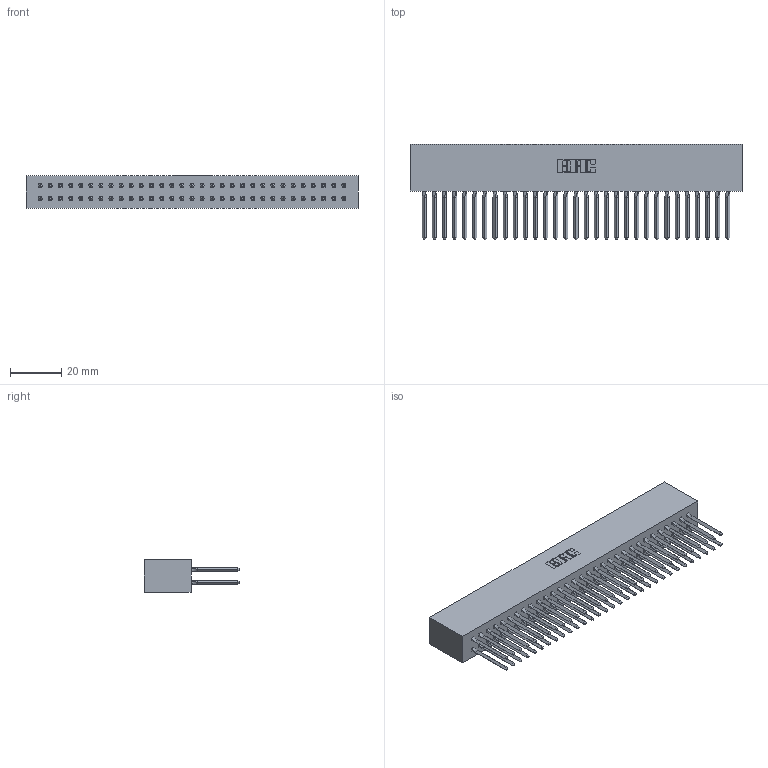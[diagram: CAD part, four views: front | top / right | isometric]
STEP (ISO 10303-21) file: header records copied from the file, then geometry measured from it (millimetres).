
FILE_DESCRIPTION (( 'STEP AP203' ), '1' );
FILE_NAME ('317-062-540-801.STEP', '2020-02-28T05:19:01', ( '' ), ( '' ), 'SwSTEP 2.0', 'SolidWorks 2016', '' );
FILE_SCHEMA (( 'CONFIG_CONTROL_DESIGN' ));
Length unit declared in the file: inch
Products named in the file (3): 317-062-540-801; 317 Part_Lugless; 317-290-001_540
Assembly tree (63 placements, depth 2):
  317-062-540-801
    317 Part_Lugless
    317-290-001_540  x62
Bounding box: 130.05 x 37.34 x 12.7 mm (x, y, z)
Volume: 23247.7 mm3; surface area: 34501.6 mm2
Topology: 63 solids, 63 shells, 5608 faces, 15553 edges, 10016 vertices
Faces by surface type: plane 4576, cylinder 784, bspline 248
Entity records: 45936 total; most frequent: CARTESIAN_POINT 8427, ORIENTED_EDGE 7926, DIRECTION 6605, EDGE_CURVE 3963, LINE 3715, VECTOR 3715, VERTEX_POINT 2635, AXIS2_PLACEMENT_3D 1445
